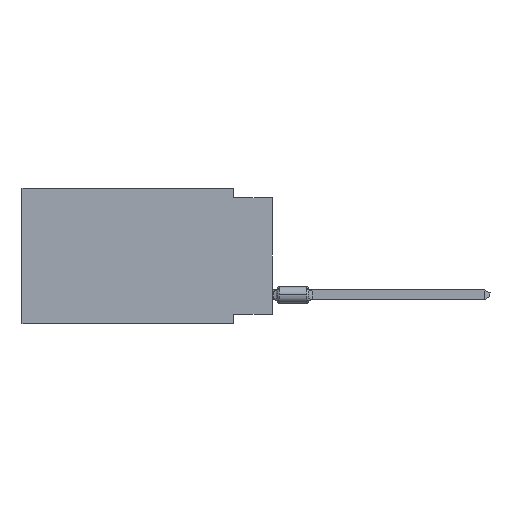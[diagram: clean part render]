
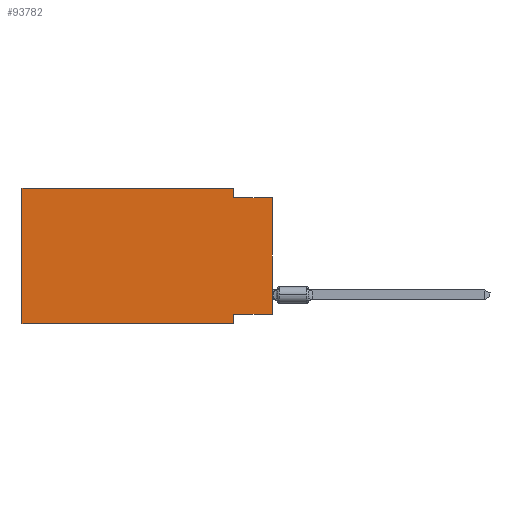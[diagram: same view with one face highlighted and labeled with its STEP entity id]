
A CAD part, left-side view. The second image highlights one B-rep face of the part: STEP entity #93782.
In plain terms, the highlighted planar face has unit normal (-1, 0, 0).
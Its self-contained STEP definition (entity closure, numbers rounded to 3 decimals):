
#2352 = EDGE_CURVE ( 'NONE', #54294, #38295, #62314, .T. ) ;
#3536 = VECTOR ( 'NONE', #78319, 1000. ) ;
#3650 = CARTESIAN_POINT ( 'NONE',  ( 0., 16.383, -8.89 ) ) ;
#3993 = EDGE_CURVE ( 'NONE', #35093, #87099, #38096, .T. ) ;
#5008 = ORIENTED_EDGE ( 'NONE', *, *, #64682, .F. ) ;
#5655 = FACE_OUTER_BOUND ( 'NONE', #28618, .T. ) ;
#5946 = CARTESIAN_POINT ( 'NONE',  ( 0., 16.383, 0. ) ) ;
#9663 = LINE ( 'NONE', #73959, #71694 ) ;
#12258 = ORIENTED_EDGE ( 'NONE', *, *, #14820, .T. ) ;
#13438 = DIRECTION ( 'NONE',  ( 0., -1., 0. ) ) ;
#14820 = EDGE_CURVE ( 'NONE', #56936, #103073, #68343, .T. ) ;
#16082 = CARTESIAN_POINT ( 'NONE',  ( 0., 0., 0. ) ) ;
#17139 = CARTESIAN_POINT ( 'NONE',  ( 0., 2.54, -8.255 ) ) ;
#19084 = LINE ( 'NONE', #100202, #55506 ) ;
#19456 = DIRECTION ( 'NONE',  ( 0., -1., 0. ) ) ;
#20118 = VERTEX_POINT ( 'NONE', #17139 ) ;
#22935 = EDGE_CURVE ( 'NONE', #56936, #20118, #9663, .T. ) ;
#24591 = DIRECTION ( 'NONE',  ( 0., 0., -1. ) ) ;
#26120 = CARTESIAN_POINT ( 'NONE',  ( 0., 2.54, -0.635 ) ) ;
#28027 = DIRECTION ( 'NONE',  ( 0., 0., -1. ) ) ;
#28437 = ORIENTED_EDGE ( 'NONE', *, *, #94153, .F. ) ;
#28618 = EDGE_LOOP ( 'NONE', ( #12258, #28437, #58524, #5008, #89492, #41081, #41738, #61303 ) ) ;
#29379 = PLANE ( 'NONE',  #59100 ) ;
#31969 = DIRECTION ( 'NONE',  ( 1., 0., 0. ) ) ;
#35093 = VERTEX_POINT ( 'NONE', #60194 ) ;
#38082 = DIRECTION ( 'NONE',  ( 0., 0., -1. ) ) ;
#38096 = LINE ( 'NONE', #62330, #44943 ) ;
#38295 = VERTEX_POINT ( 'NONE', #26120 ) ;
#41081 = ORIENTED_EDGE ( 'NONE', *, *, #48968, .T. ) ;
#41738 = ORIENTED_EDGE ( 'NONE', *, *, #44812, .F. ) ;
#42038 = CARTESIAN_POINT ( 'NONE',  ( 0., 0., -0.635 ) ) ;
#44564 = CARTESIAN_POINT ( 'NONE',  ( 0., 0., -0.635 ) ) ;
#44812 = EDGE_CURVE ( 'NONE', #20118, #49582, #19084, .T. ) ;
#44943 = VECTOR ( 'NONE', #94464, 1000. ) ;
#44972 = DIRECTION ( 'NONE',  ( 0., -1., 0. ) ) ;
#47356 = VECTOR ( 'NONE', #13438, 1000. ) ;
#48968 = EDGE_CURVE ( 'NONE', #35093, #49582, #98496, .T. ) ;
#49582 = VERTEX_POINT ( 'NONE', #80219 ) ;
#54294 = VERTEX_POINT ( 'NONE', #75994 ) ;
#55506 = VECTOR ( 'NONE', #28027, 1000. ) ;
#56936 = VERTEX_POINT ( 'NONE', #74124 ) ;
#58524 = ORIENTED_EDGE ( 'NONE', *, *, #2352, .F. ) ;
#59100 = AXIS2_PLACEMENT_3D ( 'NONE', #97299, #31969, #24591 ) ;
#60194 = CARTESIAN_POINT ( 'NONE',  ( 0., 16.383, -8.89 ) ) ;
#61303 = ORIENTED_EDGE ( 'NONE', *, *, #22935, .F. ) ;
#61829 = VECTOR ( 'NONE', #19456, 1000. ) ;
#62314 = LINE ( 'NONE', #96006, #103533 ) ;
#62330 = CARTESIAN_POINT ( 'NONE',  ( 0., 16.383, 0. ) ) ;
#64682 = EDGE_CURVE ( 'NONE', #87099, #54294, #86564, .T. ) ;
#68343 = LINE ( 'NONE', #16082, #3536 ) ;
#71694 = VECTOR ( 'NONE', #74489, 1000. ) ;
#73959 = CARTESIAN_POINT ( 'NONE',  ( 0., 0., -8.255 ) ) ;
#74124 = CARTESIAN_POINT ( 'NONE',  ( 0., 0., -8.255 ) ) ;
#74489 = DIRECTION ( 'NONE',  ( 0., 1., 0. ) ) ;
#75994 = CARTESIAN_POINT ( 'NONE',  ( 0., 2.54, 0. ) ) ;
#78319 = DIRECTION ( 'NONE',  ( 0., 0., 1. ) ) ;
#80219 = CARTESIAN_POINT ( 'NONE',  ( 0., 2.54, -8.89 ) ) ;
#81226 = CARTESIAN_POINT ( 'NONE',  ( 0., 16.383, 0. ) ) ;
#85638 = LINE ( 'NONE', #44564, #47356 ) ;
#86564 = LINE ( 'NONE', #5946, #103682 ) ;
#87099 = VERTEX_POINT ( 'NONE', #81226 ) ;
#89492 = ORIENTED_EDGE ( 'NONE', *, *, #3993, .F. ) ;
#93782 = ADVANCED_FACE ( 'NONE', ( #5655 ), #29379, .F. ) ;
#94153 = EDGE_CURVE ( 'NONE', #38295, #103073, #85638, .T. ) ;
#94464 = DIRECTION ( 'NONE',  ( 0., 0., 1. ) ) ;
#96006 = CARTESIAN_POINT ( 'NONE',  ( 0., 2.54, 0. ) ) ;
#97299 = CARTESIAN_POINT ( 'NONE',  ( 0., 16.383, 0. ) ) ;
#98496 = LINE ( 'NONE', #3650, #61829 ) ;
#100202 = CARTESIAN_POINT ( 'NONE',  ( 0., 2.54, -8.89 ) ) ;
#103073 = VERTEX_POINT ( 'NONE', #42038 ) ;
#103533 = VECTOR ( 'NONE', #38082, 1000. ) ;
#103682 = VECTOR ( 'NONE', #44972, 1000. ) ;
